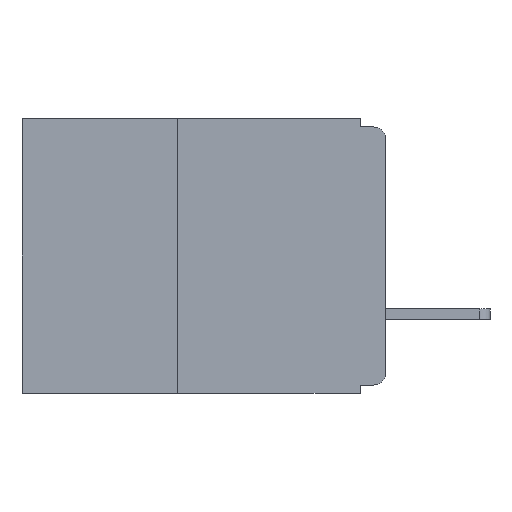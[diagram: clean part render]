
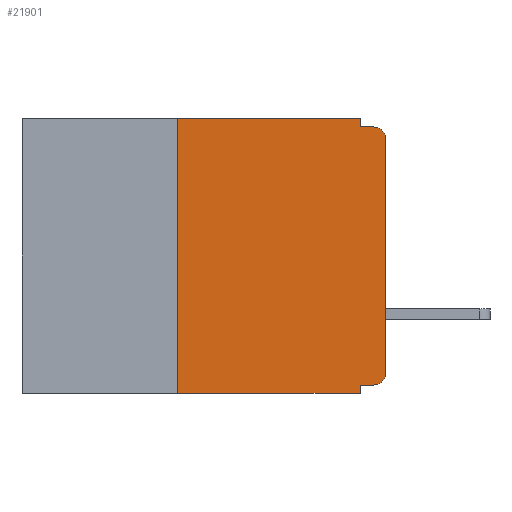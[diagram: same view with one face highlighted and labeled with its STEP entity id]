
A CAD part, left-side view. The second image highlights one B-rep face of the part: STEP entity #21901.
In plain terms, the highlighted planar face has unit normal (-1, 0, 0).
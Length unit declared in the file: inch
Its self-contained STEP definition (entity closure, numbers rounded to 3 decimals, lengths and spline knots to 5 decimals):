
#151 = EDGE_CURVE ( 'NONE', #18754, #1331, #23694, .T. ) ;
#241 = ORIENTED_EDGE ( 'NONE', *, *, #6444, .F. ) ;
#883 = DIRECTION ( 'NONE',  ( 0., 0., -1. ) ) ;
#1331 = VERTEX_POINT ( 'NONE', #10375 ) ;
#1665 = EDGE_CURVE ( 'NONE', #23470, #18754, #12777, .T. ) ;
#1986 = DIRECTION ( 'NONE',  ( 0., 1., 0. ) ) ;
#2072 = LINE ( 'NONE', #21683, #7802 ) ;
#2407 = CARTESIAN_POINT ( 'NONE',  ( 0., 0., -0.305 ) ) ;
#2491 = DIRECTION ( 'NONE',  ( 0., 0., 1. ) ) ;
#2717 = CARTESIAN_POINT ( 'NONE',  ( 0., 0.25, -0.33 ) ) ;
#3513 = LINE ( 'NONE', #16500, #15633 ) ;
#3938 = EDGE_CURVE ( 'NONE', #23470, #14484, #3513, .T. ) ;
#5262 = CARTESIAN_POINT ( 'NONE',  ( 0., 0.031, -0.32 ) ) ;
#5285 = VECTOR ( 'NONE', #12773, 39.37008 ) ;
#6360 = PLANE ( 'NONE',  #25308 ) ;
#6444 = EDGE_CURVE ( 'NONE', #23495, #14484, #18106, .T. ) ;
#6837 = CARTESIAN_POINT ( 'NONE',  ( 0., 0.031, -0.01 ) ) ;
#6841 = CARTESIAN_POINT ( 'NONE',  ( 0., 0., -0.025 ) ) ;
#7802 = VECTOR ( 'NONE', #19267, 39.37008 ) ;
#8039 = DIRECTION ( 'NONE',  ( 0., -1., 0. ) ) ;
#8757 = ORIENTED_EDGE ( 'NONE', *, *, #9458, .T. ) ;
#8837 = CARTESIAN_POINT ( 'NONE',  ( 0., 0.437, 0. ) ) ;
#8943 = VERTEX_POINT ( 'NONE', #25239 ) ;
#9458 = EDGE_CURVE ( 'NONE', #28402, #9765, #14250, .T. ) ;
#9634 = VECTOR ( 'NONE', #27731, 39.37008 ) ;
#9765 = VERTEX_POINT ( 'NONE', #2407 ) ;
#9813 = ORIENTED_EDGE ( 'NONE', *, *, #21031, .F. ) ;
#9872 = ORIENTED_EDGE ( 'NONE', *, *, #23247, .F. ) ;
#10006 = LINE ( 'NONE', #18853, #22689 ) ;
#10138 = CIRCLE ( 'NONE', #29401, 0.015 ) ;
#10375 = CARTESIAN_POINT ( 'NONE',  ( 0., 0.031, 0. ) ) ;
#10408 = EDGE_LOOP ( 'NONE', ( #21380, #24356, #13930, #9813, #15038, #17281, #17312, #241, #9872, #8757 ) ) ;
#11356 = VECTOR ( 'NONE', #2491, 39.37008 ) ;
#11377 = DIRECTION ( 'NONE',  ( -1., 0., 0. ) ) ;
#11433 = CARTESIAN_POINT ( 'NONE',  ( 0., 0.25, -0.33 ) ) ;
#11792 = VECTOR ( 'NONE', #8039, 39.37008 ) ;
#12677 = CARTESIAN_POINT ( 'NONE',  ( 0., 0.031, -0.33 ) ) ;
#12773 = DIRECTION ( 'NONE',  ( 0., 0., -1. ) ) ;
#12777 = LINE ( 'NONE', #11433, #18364 ) ;
#13049 = CARTESIAN_POINT ( 'NONE',  ( 0., 0.015, -0.32 ) ) ;
#13652 = DIRECTION ( 'NONE',  ( 0., 0., -1. ) ) ;
#13930 = ORIENTED_EDGE ( 'NONE', *, *, #22520, .F. ) ;
#14250 = CIRCLE ( 'NONE', #28581, 0.015 ) ;
#14484 = VERTEX_POINT ( 'NONE', #18325 ) ;
#14754 = EDGE_CURVE ( 'NONE', #9765, #15244, #17637, .T. ) ;
#14885 = FACE_OUTER_BOUND ( 'NONE', #10408, .T. ) ;
#15038 = ORIENTED_EDGE ( 'NONE', *, *, #151, .F. ) ;
#15244 = VERTEX_POINT ( 'NONE', #6841 ) ;
#15413 = DIRECTION ( 'NONE',  ( -1., 0., 0. ) ) ;
#15633 = VECTOR ( 'NONE', #16408, 39.37008 ) ;
#16408 = DIRECTION ( 'NONE',  ( 0., -1., 0. ) ) ;
#16500 = CARTESIAN_POINT ( 'NONE',  ( 0., 0.437, -0.33 ) ) ;
#16940 = CARTESIAN_POINT ( 'NONE',  ( 0., 0., 0. ) ) ;
#17281 = ORIENTED_EDGE ( 'NONE', *, *, #1665, .F. ) ;
#17312 = ORIENTED_EDGE ( 'NONE', *, *, #3938, .T. ) ;
#17637 = LINE ( 'NONE', #16940, #11356 ) ;
#18106 = LINE ( 'NONE', #12677, #5285 ) ;
#18325 = CARTESIAN_POINT ( 'NONE',  ( 0., 0.031, -0.33 ) ) ;
#18364 = VECTOR ( 'NONE', #26596, 39.37008 ) ;
#18754 = VERTEX_POINT ( 'NONE', #22128 ) ;
#18853 = CARTESIAN_POINT ( 'NONE',  ( 0., 0., -0.32 ) ) ;
#19267 = DIRECTION ( 'NONE',  ( 0., 0., -1. ) ) ;
#21031 = EDGE_CURVE ( 'NONE', #1331, #29903, #2072, .T. ) ;
#21260 = LINE ( 'NONE', #25368, #9634 ) ;
#21380 = ORIENTED_EDGE ( 'NONE', *, *, #14754, .T. ) ;
#21683 = CARTESIAN_POINT ( 'NONE',  ( 0., 0.031, 0. ) ) ;
#21901 = ADVANCED_FACE ( 'NONE', ( #14885 ), #6360, .F. ) ;
#22128 = CARTESIAN_POINT ( 'NONE',  ( 0., 0.25, 0. ) ) ;
#22520 = EDGE_CURVE ( 'NONE', #29903, #8943, #21260, .T. ) ;
#22689 = VECTOR ( 'NONE', #1986, 39.37008 ) ;
#23247 = EDGE_CURVE ( 'NONE', #28402, #23495, #10006, .T. ) ;
#23470 = VERTEX_POINT ( 'NONE', #2717 ) ;
#23495 = VERTEX_POINT ( 'NONE', #5262 ) ;
#23694 = LINE ( 'NONE', #25456, #11792 ) ;
#23758 = EDGE_CURVE ( 'NONE', #15244, #8943, #10138, .T. ) ;
#24356 = ORIENTED_EDGE ( 'NONE', *, *, #23758, .T. ) ;
#25239 = CARTESIAN_POINT ( 'NONE',  ( 0., 0.015, -0.01 ) ) ;
#25308 = AXIS2_PLACEMENT_3D ( 'NONE', #8837, #27868, #13652 ) ;
#25368 = CARTESIAN_POINT ( 'NONE',  ( 0., 0., -0.01 ) ) ;
#25456 = CARTESIAN_POINT ( 'NONE',  ( 0., 0.437, 0. ) ) ;
#25611 = CARTESIAN_POINT ( 'NONE',  ( 0., 0.015, -0.025 ) ) ;
#26596 = DIRECTION ( 'NONE',  ( 0., 0., 1. ) ) ;
#27731 = DIRECTION ( 'NONE',  ( 0., -1., 0. ) ) ;
#27868 = DIRECTION ( 'NONE',  ( 1., 0., 0. ) ) ;
#27959 = DIRECTION ( 'NONE',  ( 0., 0., -1. ) ) ;
#28402 = VERTEX_POINT ( 'NONE', #13049 ) ;
#28581 = AXIS2_PLACEMENT_3D ( 'NONE', #29588, #15413, #883 ) ;
#29401 = AXIS2_PLACEMENT_3D ( 'NONE', #25611, #11377, #27959 ) ;
#29588 = CARTESIAN_POINT ( 'NONE',  ( 0., 0.015, -0.305 ) ) ;
#29903 = VERTEX_POINT ( 'NONE', #6837 ) ;
